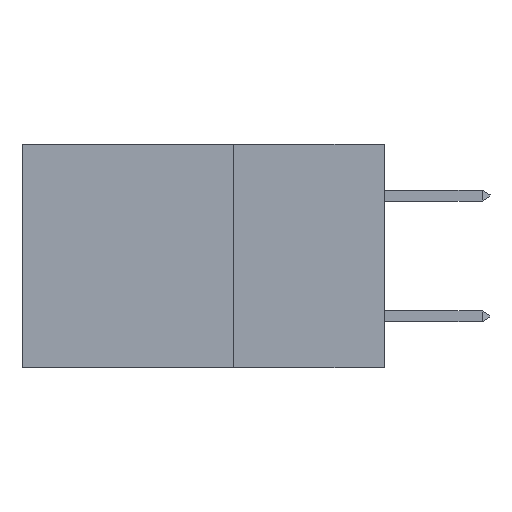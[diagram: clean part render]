
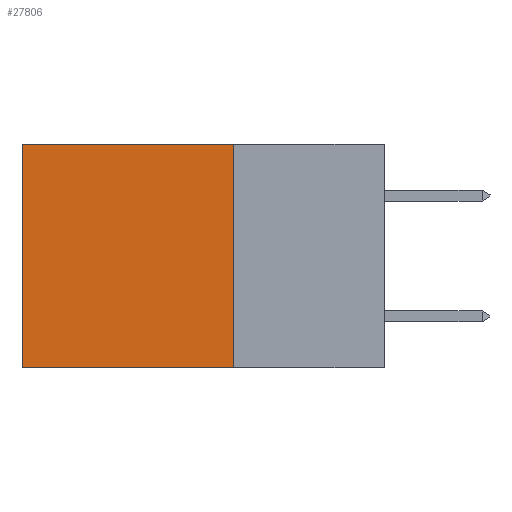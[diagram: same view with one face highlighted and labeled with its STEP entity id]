
A CAD part, left-side view. The second image highlights one B-rep face of the part: STEP entity #27806.
In plain terms, the highlighted planar face has unit normal (-1, 0, 0).
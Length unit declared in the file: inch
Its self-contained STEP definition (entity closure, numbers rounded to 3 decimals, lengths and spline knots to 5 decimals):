
#586 = FACE_OUTER_BOUND ( 'NONE', #1849, .T. ) ;
#1839 = CARTESIAN_POINT ( 'NONE',  ( 0.2875, 0.25, -0.37 ) ) ;
#1849 = EDGE_LOOP ( 'NONE', ( #22773, #8397, #12927, #8714 ) ) ;
#3479 = CARTESIAN_POINT ( 'NONE',  ( 0.2875, 0.6, 0. ) ) ;
#3724 = CARTESIAN_POINT ( 'NONE',  ( 0.2875, 0.25, -0.37 ) ) ;
#5360 = EDGE_CURVE ( 'NONE', #7070, #22089, #22122, .T. ) ;
#5749 = DIRECTION ( 'NONE',  ( 0., 0., -1. ) ) ;
#7070 = VERTEX_POINT ( 'NONE', #3479 ) ;
#7128 = VECTOR ( 'NONE', #14626, 39.37008 ) ;
#8261 = CARTESIAN_POINT ( 'NONE',  ( 0.2875, 0.6, 0. ) ) ;
#8397 = ORIENTED_EDGE ( 'NONE', *, *, #25331, .F. ) ;
#8714 = ORIENTED_EDGE ( 'NONE', *, *, #19127, .T. ) ;
#9575 = CARTESIAN_POINT ( 'NONE',  ( 0.2875, 0.25, 0. ) ) ;
#12425 = VECTOR ( 'NONE', #19542, 39.37008 ) ;
#12927 = ORIENTED_EDGE ( 'NONE', *, *, #13243, .F. ) ;
#13243 = EDGE_CURVE ( 'NONE', #22996, #17310, #21293, .T. ) ;
#14626 = DIRECTION ( 'NONE',  ( 0., 0., -1. ) ) ;
#15440 = CARTESIAN_POINT ( 'NONE',  ( 0.2875, 0.6, -0.37 ) ) ;
#16801 = VECTOR ( 'NONE', #18853, 39.37008 ) ;
#17256 = CARTESIAN_POINT ( 'NONE',  ( 0.2875, 0.25, 0. ) ) ;
#17293 = DIRECTION ( 'NONE',  ( 0., 0., -1. ) ) ;
#17310 = VERTEX_POINT ( 'NONE', #1839 ) ;
#18853 = DIRECTION ( 'NONE',  ( 0., 1., 0. ) ) ;
#19127 = EDGE_CURVE ( 'NONE', #22996, #7070, #21071, .T. ) ;
#19465 = CARTESIAN_POINT ( 'NONE',  ( 0.2875, 0.25, 0. ) ) ;
#19542 = DIRECTION ( 'NONE',  ( 0., 1., 0. ) ) ;
#21071 = LINE ( 'NONE', #9575, #16801 ) ;
#21293 = LINE ( 'NONE', #17256, #7128 ) ;
#22089 = VERTEX_POINT ( 'NONE', #15440 ) ;
#22122 = LINE ( 'NONE', #8261, #24234 ) ;
#22773 = ORIENTED_EDGE ( 'NONE', *, *, #5360, .T. ) ;
#22996 = VERTEX_POINT ( 'NONE', #28068 ) ;
#23539 = AXIS2_PLACEMENT_3D ( 'NONE', #19465, #28239, #5749 ) ;
#24234 = VECTOR ( 'NONE', #17293, 39.37008 ) ;
#25331 = EDGE_CURVE ( 'NONE', #17310, #22089, #29020, .T. ) ;
#26268 = PLANE ( 'NONE',  #23539 ) ;
#27806 = ADVANCED_FACE ( 'NONE', ( #586 ), #26268, .F. ) ;
#28068 = CARTESIAN_POINT ( 'NONE',  ( 0.2875, 0.25, 0. ) ) ;
#28239 = DIRECTION ( 'NONE',  ( 1., 0., 0. ) ) ;
#29020 = LINE ( 'NONE', #3724, #12425 ) ;
